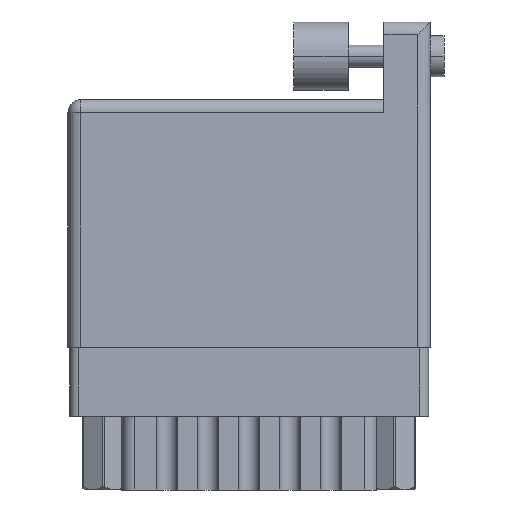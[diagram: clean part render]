
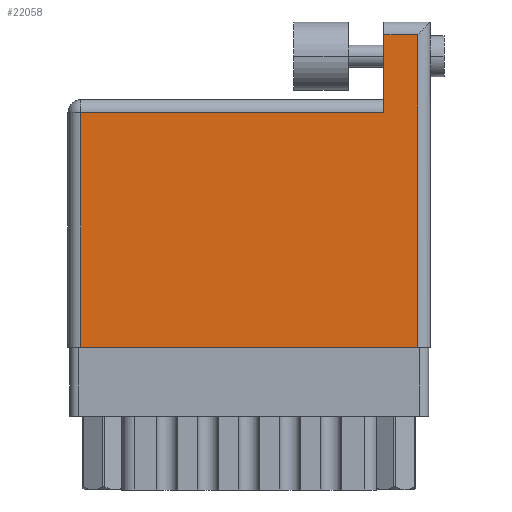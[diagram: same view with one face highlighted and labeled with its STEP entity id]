
A CAD part, front view. The second image highlights one B-rep face of the part: STEP entity #22058.
In plain terms, the highlighted face is planar.
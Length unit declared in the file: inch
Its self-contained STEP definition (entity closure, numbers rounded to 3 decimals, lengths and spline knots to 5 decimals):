
#822 = CARTESIAN_POINT ( 'NONE',  ( 1.155, 0.859, 0. ) ) ;
#883 = DIRECTION ( 'NONE',  ( -1., 0., 0. ) ) ;
#3514 = LINE ( 'NONE', #16838, #24445 ) ;
#4007 = VERTEX_POINT ( 'NONE', #822 ) ;
#4500 = CARTESIAN_POINT ( 'NONE',  ( 0., 0.859, 0. ) ) ;
#4670 = CARTESIAN_POINT ( 'NONE',  ( 1.155, 1.143, 0. ) ) ;
#5297 = CARTESIAN_POINT ( 'NONE',  ( 1.155, 1.19, 0. ) ) ;
#5818 = VERTEX_POINT ( 'NONE', #13262 ) ;
#6010 = VERTEX_POINT ( 'NONE', #16424 ) ;
#6326 = CARTESIAN_POINT ( 'NONE',  ( 0., 0., 0. ) ) ;
#6759 = VECTOR ( 'NONE', #15376, 39.37008 ) ;
#6812 = DIRECTION ( 'NONE',  ( -1., 0., 0. ) ) ;
#6854 = VECTOR ( 'NONE', #19632, 39.37008 ) ;
#6975 = LINE ( 'NONE', #4670, #6759 ) ;
#7892 = VECTOR ( 'NONE', #15735, 39.37008 ) ;
#8605 = DIRECTION ( 'NONE',  ( 0., 0., -1. ) ) ;
#9262 = ORIENTED_EDGE ( 'NONE', *, *, #28269, .T. ) ;
#9279 = DIRECTION ( 'NONE',  ( 0., -1., 0. ) ) ;
#9522 = ORIENTED_EDGE ( 'NONE', *, *, #19217, .T. ) ;
#10381 = CARTESIAN_POINT ( 'NONE',  ( 1.278, 1.143, 0. ) ) ;
#11919 = LINE ( 'NONE', #6326, #6854 ) ;
#13025 = DIRECTION ( 'NONE',  ( 0., -1., 0. ) ) ;
#13262 = CARTESIAN_POINT ( 'NONE',  ( 1.278, 0., 0. ) ) ;
#13402 = CARTESIAN_POINT ( 'NONE',  ( 1.155, 1.143, 0. ) ) ;
#13651 = VERTEX_POINT ( 'NONE', #10381 ) ;
#13803 = EDGE_LOOP ( 'NONE', ( #15931, #9522, #30783, #30196, #29289, #9262 ) ) ;
#13996 = VECTOR ( 'NONE', #13025, 39.37008 ) ;
#15152 = VECTOR ( 'NONE', #6812, 39.37008 ) ;
#15376 = DIRECTION ( 'NONE',  ( -1., 0., 0. ) ) ;
#15735 = DIRECTION ( 'NONE',  ( 0., 1., 0. ) ) ;
#15931 = ORIENTED_EDGE ( 'NONE', *, *, #16008, .T. ) ;
#16008 = EDGE_CURVE ( 'NONE', #23124, #5818, #11919, .T. ) ;
#16166 = PLANE ( 'NONE',  #18478 ) ;
#16424 = CARTESIAN_POINT ( 'NONE',  ( 0.047, 0.859, 0. ) ) ;
#16838 = CARTESIAN_POINT ( 'NONE',  ( 0.047, 0., 0. ) ) ;
#17829 = LINE ( 'NONE', #20973, #7892 ) ;
#18084 = EDGE_CURVE ( 'NONE', #19964, #4007, #26487, .T. ) ;
#18478 = AXIS2_PLACEMENT_3D ( 'NONE', #32579, #8605, #883 ) ;
#18966 = FACE_OUTER_BOUND ( 'NONE', #13803, .T. ) ;
#19217 = EDGE_CURVE ( 'NONE', #5818, #13651, #17829, .T. ) ;
#19632 = DIRECTION ( 'NONE',  ( 1., 0., 0. ) ) ;
#19964 = VERTEX_POINT ( 'NONE', #13402 ) ;
#20668 = EDGE_CURVE ( 'NONE', #4007, #6010, #25358, .T. ) ;
#20755 = EDGE_CURVE ( 'NONE', #13651, #19964, #6975, .T. ) ;
#20973 = CARTESIAN_POINT ( 'NONE',  ( 1.278, 1.19, 0. ) ) ;
#22058 = ADVANCED_FACE ( 'NONE', ( #18966 ), #16166, .F. ) ;
#23124 = VERTEX_POINT ( 'NONE', #25575 ) ;
#24445 = VECTOR ( 'NONE', #9279, 39.37008 ) ;
#25358 = LINE ( 'NONE', #4500, #15152 ) ;
#25575 = CARTESIAN_POINT ( 'NONE',  ( 0.047, 0., 0. ) ) ;
#26487 = LINE ( 'NONE', #5297, #13996 ) ;
#28269 = EDGE_CURVE ( 'NONE', #6010, #23124, #3514, .T. ) ;
#29289 = ORIENTED_EDGE ( 'NONE', *, *, #20668, .T. ) ;
#30196 = ORIENTED_EDGE ( 'NONE', *, *, #18084, .T. ) ;
#30783 = ORIENTED_EDGE ( 'NONE', *, *, #20755, .T. ) ;
#32579 = CARTESIAN_POINT ( 'NONE',  ( 0., 0.906, 0. ) ) ;
